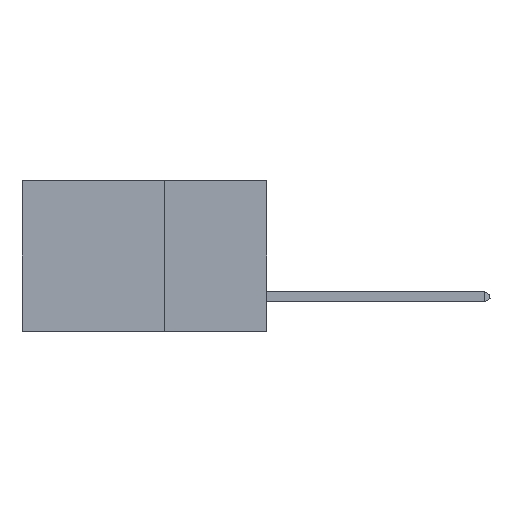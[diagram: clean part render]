
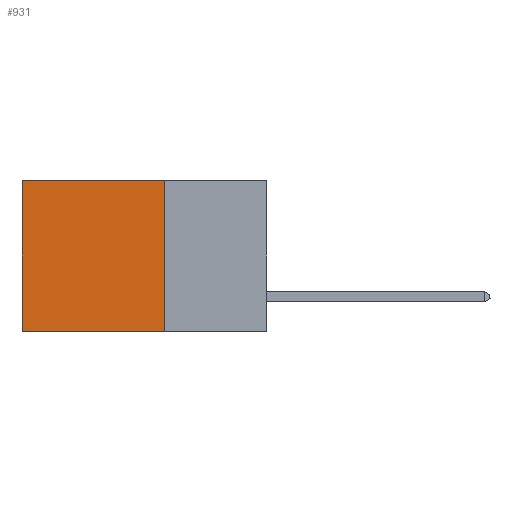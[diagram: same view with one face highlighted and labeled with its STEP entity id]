
A CAD part, left-side view. The second image highlights one B-rep face of the part: STEP entity #931.
In plain terms, the highlighted planar face has unit normal (-1, 0, 0).
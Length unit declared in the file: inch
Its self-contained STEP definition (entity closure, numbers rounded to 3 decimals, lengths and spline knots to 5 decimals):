
#210 = CARTESIAN_POINT ( 'NONE',  ( 0.2875, 0.25, -0.37 ) ) ;
#931 = ADVANCED_FACE ( 'NONE', ( #39238 ), #10103, .F. ) ;
#2441 = LINE ( 'NONE', #210, #27796 ) ;
#3012 = CARTESIAN_POINT ( 'NONE',  ( 0.2875, 0.25, 0. ) ) ;
#4611 = CARTESIAN_POINT ( 'NONE',  ( 0.2875, 0.25, -0.37 ) ) ;
#5055 = CARTESIAN_POINT ( 'NONE',  ( 0.2875, 0.6, 0. ) ) ;
#8256 = DIRECTION ( 'NONE',  ( 0., 0., -1. ) ) ;
#10103 = PLANE ( 'NONE',  #13156 ) ;
#11070 = DIRECTION ( 'NONE',  ( 0., 1., 0. ) ) ;
#13156 = AXIS2_PLACEMENT_3D ( 'NONE', #3012, #34182, #26729 ) ;
#13893 = LINE ( 'NONE', #28391, #25289 ) ;
#18300 = CARTESIAN_POINT ( 'NONE',  ( 0.2875, 0.6, 0. ) ) ;
#18559 = EDGE_CURVE ( 'NONE', #23620, #19020, #13893, .T. ) ;
#19020 = VERTEX_POINT ( 'NONE', #4611 ) ;
#20620 = ORIENTED_EDGE ( 'NONE', *, *, #24868, .T. ) ;
#22989 = EDGE_LOOP ( 'NONE', ( #20620, #34730, #33684, #27734 ) ) ;
#23202 = DIRECTION ( 'NONE',  ( 0., 1., 0. ) ) ;
#23620 = VERTEX_POINT ( 'NONE', #28930 ) ;
#24868 = EDGE_CURVE ( 'NONE', #31373, #35967, #41456, .T. ) ;
#25168 = LINE ( 'NONE', #36735, #43944 ) ;
#25289 = VECTOR ( 'NONE', #42471, 39.37008 ) ;
#26729 = DIRECTION ( 'NONE',  ( 0., 0., -1. ) ) ;
#27734 = ORIENTED_EDGE ( 'NONE', *, *, #40228, .T. ) ;
#27796 = VECTOR ( 'NONE', #11070, 39.37008 ) ;
#28391 = CARTESIAN_POINT ( 'NONE',  ( 0.2875, 0.25, 0. ) ) ;
#28930 = CARTESIAN_POINT ( 'NONE',  ( 0.2875, 0.25, 0. ) ) ;
#31373 = VERTEX_POINT ( 'NONE', #5055 ) ;
#33684 = ORIENTED_EDGE ( 'NONE', *, *, #18559, .F. ) ;
#34182 = DIRECTION ( 'NONE',  ( 1., 0., 0. ) ) ;
#34730 = ORIENTED_EDGE ( 'NONE', *, *, #42169, .F. ) ;
#35967 = VERTEX_POINT ( 'NONE', #41808 ) ;
#36735 = CARTESIAN_POINT ( 'NONE',  ( 0.2875, 0.25, 0. ) ) ;
#39238 = FACE_OUTER_BOUND ( 'NONE', #22989, .T. ) ;
#40228 = EDGE_CURVE ( 'NONE', #23620, #31373, #25168, .T. ) ;
#40395 = VECTOR ( 'NONE', #8256, 39.37008 ) ;
#41456 = LINE ( 'NONE', #18300, #40395 ) ;
#41808 = CARTESIAN_POINT ( 'NONE',  ( 0.2875, 0.6, -0.37 ) ) ;
#42169 = EDGE_CURVE ( 'NONE', #19020, #35967, #2441, .T. ) ;
#42471 = DIRECTION ( 'NONE',  ( 0., 0., -1. ) ) ;
#43944 = VECTOR ( 'NONE', #23202, 39.37008 ) ;
